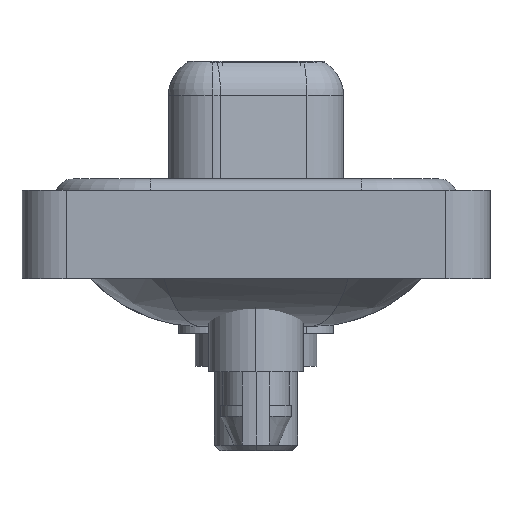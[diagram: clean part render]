
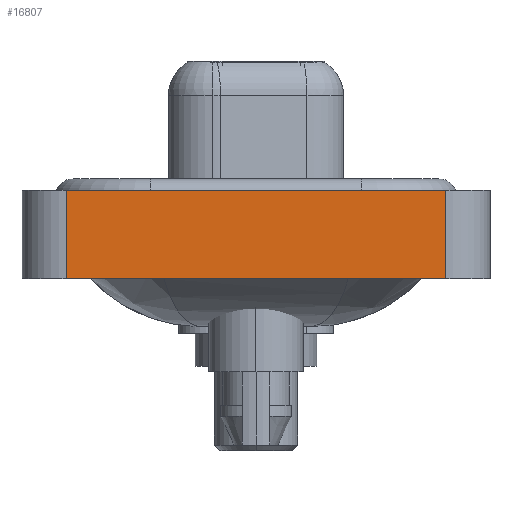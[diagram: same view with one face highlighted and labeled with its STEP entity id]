
A CAD part, left-side view. The second image highlights one B-rep face of the part: STEP entity #16807.
In plain terms, the highlighted planar face has unit normal (-1, 0, 0).
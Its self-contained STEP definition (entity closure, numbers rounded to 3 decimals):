
#152 = CARTESIAN_POINT ( 'NONE',  ( -7.25, 8.55, -3.6 ) ) ;
#331 = EDGE_LOOP ( 'NONE', ( #15723, #6013, #17512, #2119 ) ) ;
#622 = VECTOR ( 'NONE', #4354, 1000. ) ;
#2119 = ORIENTED_EDGE ( 'NONE', *, *, #7136, .T. ) ;
#2531 = CARTESIAN_POINT ( 'NONE',  ( -7.25, 8.55, 0.4 ) ) ;
#3004 = LINE ( 'NONE', #8440, #8281 ) ;
#4256 = DIRECTION ( 'NONE',  ( 0., -1., 0. ) ) ;
#4354 = DIRECTION ( 'NONE',  ( 0., 0., 1. ) ) ;
#4798 = DIRECTION ( 'NONE',  ( 0., 0., 1. ) ) ;
#5184 = AXIS2_PLACEMENT_3D ( 'NONE', #14326, #17187, #4798 ) ;
#5573 = EDGE_CURVE ( 'NONE', #14874, #15726, #7848, .T. ) ;
#6013 = ORIENTED_EDGE ( 'NONE', *, *, #5573, .F. ) ;
#6574 = VECTOR ( 'NONE', #7530, 1000. ) ;
#7136 = EDGE_CURVE ( 'NONE', #11878, #7505, #3004, .T. ) ;
#7505 = VERTEX_POINT ( 'NONE', #11801 ) ;
#7530 = DIRECTION ( 'NONE',  ( 0., 0., 1. ) ) ;
#7848 = LINE ( 'NONE', #17480, #9675 ) ;
#8260 = CARTESIAN_POINT ( 'NONE',  ( -7.25, -8.55, 0.4 ) ) ;
#8281 = VECTOR ( 'NONE', #4256, 1000. ) ;
#8440 = CARTESIAN_POINT ( 'NONE',  ( -7.25, -8.55, -3.6 ) ) ;
#9675 = VECTOR ( 'NONE', #14431, 1000. ) ;
#10349 = PLANE ( 'NONE',  #5184 ) ;
#11472 = CARTESIAN_POINT ( 'NONE',  ( -7.25, 8.55, -3.6 ) ) ;
#11801 = CARTESIAN_POINT ( 'NONE',  ( -7.25, -8.55, -3.6 ) ) ;
#11878 = VERTEX_POINT ( 'NONE', #152 ) ;
#12374 = CARTESIAN_POINT ( 'NONE',  ( -7.25, -8.55, -3.6 ) ) ;
#13081 = FACE_OUTER_BOUND ( 'NONE', #331, .T. ) ;
#14268 = EDGE_CURVE ( 'NONE', #7505, #15726, #16554, .T. ) ;
#14326 = CARTESIAN_POINT ( 'NONE',  ( -7.25, -8.55, -3.6 ) ) ;
#14431 = DIRECTION ( 'NONE',  ( 0., -1., 0. ) ) ;
#14874 = VERTEX_POINT ( 'NONE', #2531 ) ;
#15365 = LINE ( 'NONE', #11472, #6574 ) ;
#15723 = ORIENTED_EDGE ( 'NONE', *, *, #14268, .T. ) ;
#15726 = VERTEX_POINT ( 'NONE', #8260 ) ;
#15856 = EDGE_CURVE ( 'NONE', #11878, #14874, #15365, .T. ) ;
#16554 = LINE ( 'NONE', #12374, #622 ) ;
#16807 = ADVANCED_FACE ( 'NONE', ( #13081 ), #10349, .T. ) ;
#17187 = DIRECTION ( 'NONE',  ( -1., 0., 0. ) ) ;
#17480 = CARTESIAN_POINT ( 'NONE',  ( -7.25, -8.55, 0.4 ) ) ;
#17512 = ORIENTED_EDGE ( 'NONE', *, *, #15856, .F. ) ;
